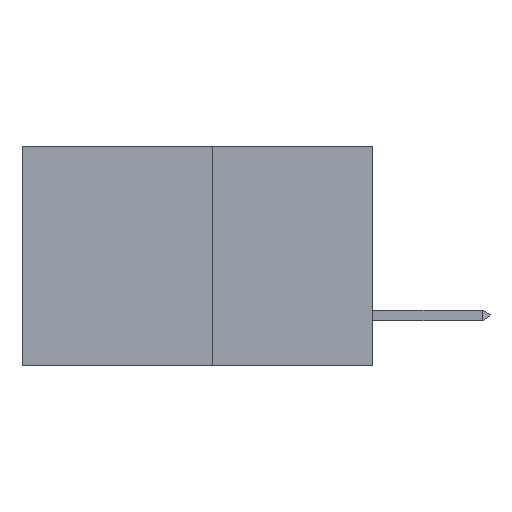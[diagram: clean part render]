
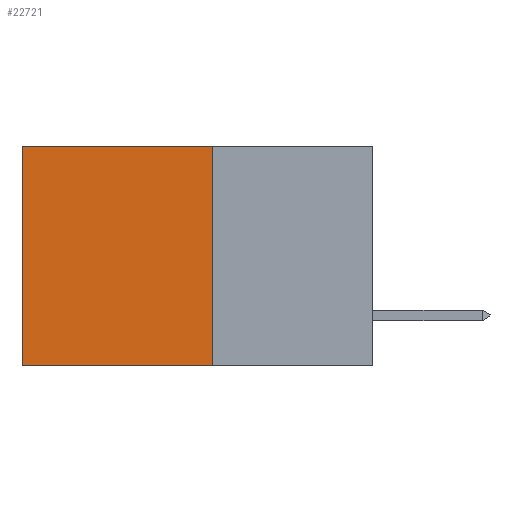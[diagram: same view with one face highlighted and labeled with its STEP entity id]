
A CAD part, left-side view. The second image highlights one B-rep face of the part: STEP entity #22721.
In plain terms, the highlighted planar face has unit normal (-1, 0, 0).
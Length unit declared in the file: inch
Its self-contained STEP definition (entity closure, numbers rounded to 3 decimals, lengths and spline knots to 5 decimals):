
#1184 = ORIENTED_EDGE ( 'NONE', *, *, #12868, .F. ) ;
#1676 = CARTESIAN_POINT ( 'NONE',  ( 0.277, 0.27, -0.37 ) ) ;
#2800 = LINE ( 'NONE', #17236, #12968 ) ;
#3268 = VECTOR ( 'NONE', #14147, 39.37008 ) ;
#3531 = VERTEX_POINT ( 'NONE', #10757 ) ;
#3576 = CARTESIAN_POINT ( 'NONE',  ( 0.277, 0.27, 0. ) ) ;
#4538 = CARTESIAN_POINT ( 'NONE',  ( 0.277, 0.59, -0.37 ) ) ;
#4893 = VERTEX_POINT ( 'NONE', #9553 ) ;
#5234 = VERTEX_POINT ( 'NONE', #20699 ) ;
#5524 = DIRECTION ( 'NONE',  ( 0., 1., 0. ) ) ;
#5927 = DIRECTION ( 'NONE',  ( 0., 0., -1. ) ) ;
#6381 = FACE_OUTER_BOUND ( 'NONE', #7568, .T. ) ;
#6595 = ORIENTED_EDGE ( 'NONE', *, *, #14430, .T. ) ;
#7190 = CARTESIAN_POINT ( 'NONE',  ( 0.277, 0.27, 0. ) ) ;
#7568 = EDGE_LOOP ( 'NONE', ( #6595, #1184, #10896, #7924 ) ) ;
#7703 = VERTEX_POINT ( 'NONE', #3576 ) ;
#7836 = PLANE ( 'NONE',  #18526 ) ;
#7924 = ORIENTED_EDGE ( 'NONE', *, *, #15411, .T. ) ;
#9553 = CARTESIAN_POINT ( 'NONE',  ( 0.277, 0.27, -0.37 ) ) ;
#9756 = CARTESIAN_POINT ( 'NONE',  ( 0.277, 0.27, -0.37 ) ) ;
#10005 = VECTOR ( 'NONE', #5524, 39.37008 ) ;
#10757 = CARTESIAN_POINT ( 'NONE',  ( 0.277, 0.59, -0.37 ) ) ;
#10896 = ORIENTED_EDGE ( 'NONE', *, *, #12350, .F. ) ;
#12350 = EDGE_CURVE ( 'NONE', #7703, #4893, #2800, .T. ) ;
#12868 = EDGE_CURVE ( 'NONE', #4893, #3531, #20668, .T. ) ;
#12968 = VECTOR ( 'NONE', #19187, 39.37008 ) ;
#14147 = DIRECTION ( 'NONE',  ( 0., 0., -1. ) ) ;
#14430 = EDGE_CURVE ( 'NONE', #5234, #3531, #19038, .T. ) ;
#15411 = EDGE_CURVE ( 'NONE', #7703, #5234, #23823, .T. ) ;
#17236 = CARTESIAN_POINT ( 'NONE',  ( 0.277, 0.27, -0.37 ) ) ;
#17287 = DIRECTION ( 'NONE',  ( 1., 0., 0. ) ) ;
#18526 = AXIS2_PLACEMENT_3D ( 'NONE', #9756, #17287, #5927 ) ;
#18692 = VECTOR ( 'NONE', #24335, 39.37008 ) ;
#19038 = LINE ( 'NONE', #4538, #3268 ) ;
#19187 = DIRECTION ( 'NONE',  ( 0., 0., -1. ) ) ;
#20668 = LINE ( 'NONE', #1676, #10005 ) ;
#20699 = CARTESIAN_POINT ( 'NONE',  ( 0.277, 0.59, 0. ) ) ;
#22721 = ADVANCED_FACE ( 'NONE', ( #6381 ), #7836, .F. ) ;
#23823 = LINE ( 'NONE', #7190, #18692 ) ;
#24335 = DIRECTION ( 'NONE',  ( 0., 1., 0. ) ) ;
